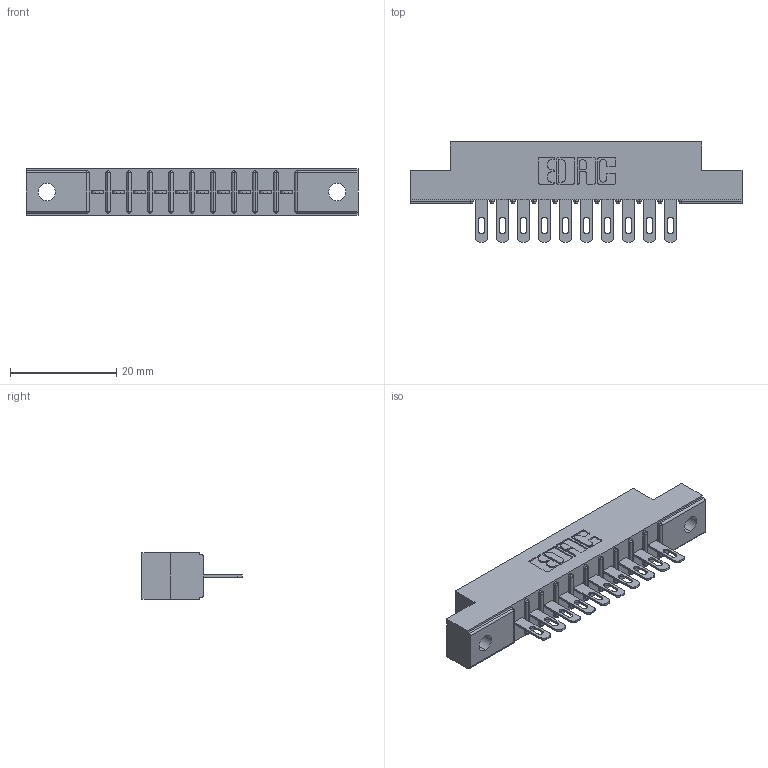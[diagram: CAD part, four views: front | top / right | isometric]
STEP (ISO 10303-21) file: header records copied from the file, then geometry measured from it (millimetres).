
FILE_DESCRIPTION (( 'STEP AP203' ), '1' );
FILE_NAME ('316-010-500-102.STEP', '2018-07-31T00:04:45', ( '' ), ( '' ), 'SwSTEP 2.0', 'SolidWorks 2016', '' );
FILE_SCHEMA (( 'CONFIG_CONTROL_DESIGN' ));
Length unit declared in the file: inch
Products named in the file (3): 306 Part_.128 Dia; 306-290-001_100; 316-010-500-102
Assembly tree (11 placements, depth 2):
  316-010-500-102
    306 Part_.128 Dia
    306-290-001_100  x10
Bounding box: 62.64 x 18.87 x 8.71 mm (x, y, z)
Volume: 4230.4 mm3; surface area: 5764.9 mm2
Topology: 11 solids, 11 shells, 876 faces, 2466 edges, 1588 vertices
Faces by surface type: plane 568, cylinder 268, sphere 40
Entity records: 13637 total; most frequent: CARTESIAN_POINT 2285, ORIENTED_EDGE 2260, DIRECTION 2258, EDGE_CURVE 1130, VECTOR 864, LINE 864, VERTEX_POINT 724, AXIS2_PLACEMENT_3D 697
